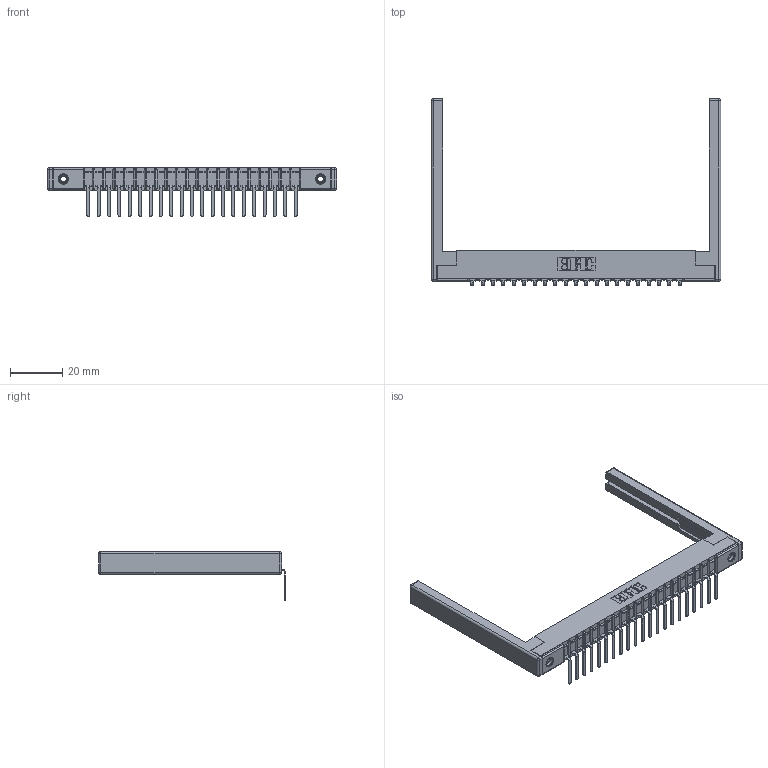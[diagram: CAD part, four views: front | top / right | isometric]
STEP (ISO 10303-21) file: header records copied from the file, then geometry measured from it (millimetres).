
FILE_DESCRIPTION (( 'STEP AP203' ), '1' );
FILE_NAME ('357-021-557-168.STEP', '2019-09-16T23:01:29', ( '' ), ( '' ), 'SwSTEP 2.0', 'SolidWorks 2016', '' );
FILE_SCHEMA (( 'CONFIG_CONTROL_DESIGN' ));
Length unit declared in the file: inch
Products named in the file (5): 307-220-068; 307 Part_.156 Dia Mounting Holes; 357-021-557-168; 307-290-002_557; 345-250-001_345-250-001-102
Assembly tree (26 placements, depth 2):
  357-021-557-168
    307 Part_.156 Dia Mounting Holes
    307-290-002_557  x21
    307-220-068  x2
    345-250-001_345-250-001-102  x2
Bounding box: 110.64 x 71.29 x 18.67 mm (x, y, z)
Volume: 11919.3 mm3; surface area: 17698.8 mm2
Topology: 26 solids, 26 shells, 1932 faces, 5837 edges, 3810 vertices
Faces by surface type: plane 1145, cylinder 719, sphere 52, cone 12, torus 4
Entity records: 24205 total; most frequent: CARTESIAN_POINT 4045, ORIENTED_EDGE 4024, DIRECTION 3958, EDGE_CURVE 2012, LINE 1528, VECTOR 1528, VERTEX_POINT 1302, AXIS2_PLACEMENT_3D 1215
